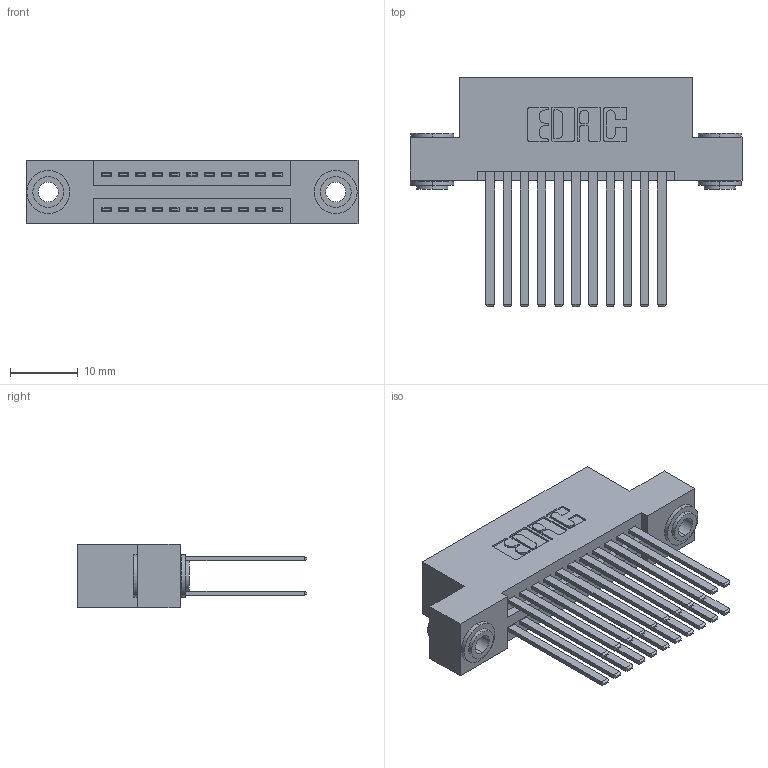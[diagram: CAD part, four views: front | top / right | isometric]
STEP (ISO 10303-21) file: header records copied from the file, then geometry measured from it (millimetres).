
FILE_DESCRIPTION (( 'STEP AP203' ), '1' );
FILE_NAME ('395-022-544-203.STEP', '2018-11-08T04:32:38', ( '' ), ( '' ), 'SwSTEP 2.0', 'SolidWorks 2016', '' );
FILE_SCHEMA (( 'CONFIG_CONTROL_DESIGN' ));
Length unit declared in the file: inch
Products named in the file (4): 345 Part_Flush Mounting Lugs - 0.156 Dia-TH; 395-022-544-203; 345-250-002_345-250-002-102; 345-292-001_345-293-144
Assembly tree (25 placements, depth 2):
  395-022-544-203
    345 Part_Flush Mounting Lugs - 0.156 Dia-TH
    345-292-001_345-293-144  x22
    345-250-002_345-250-002-102  x2
Bounding box: 49.15 x 33.96 x 9.4 mm (x, y, z)
Volume: 4814.4 mm3; surface area: 7624.9 mm2
Topology: 25 solids, 25 shells, 1132 faces, 3299 edges, 2166 vertices
Faces by surface type: plane 728, cylinder 396, cone 8
Entity records: 13270 total; most frequent: CARTESIAN_POINT 2227, ORIENTED_EDGE 2154, DIRECTION 2031, EDGE_CURVE 1077, VECTOR 881, LINE 881, VERTEX_POINT 714, AXIS2_PLACEMENT_3D 575
